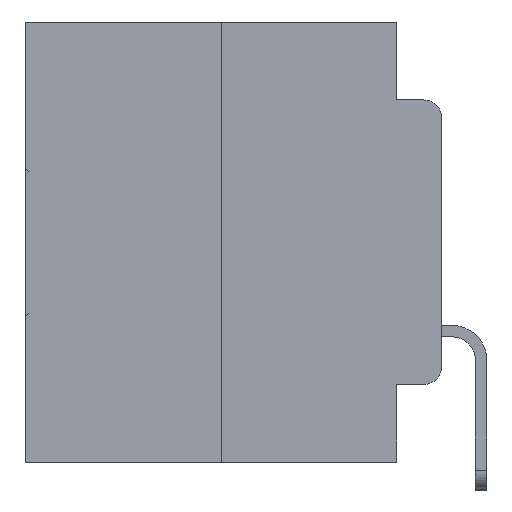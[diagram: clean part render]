
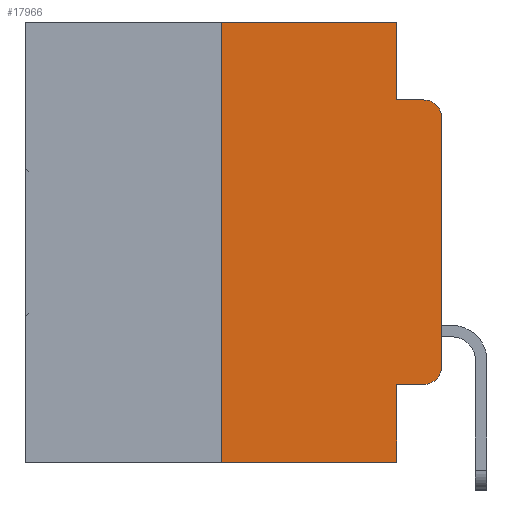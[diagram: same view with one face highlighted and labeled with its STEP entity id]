
A CAD part, left-side view. The second image highlights one B-rep face of the part: STEP entity #17966.
In plain terms, the highlighted planar face has unit normal (-1, 0, 0).
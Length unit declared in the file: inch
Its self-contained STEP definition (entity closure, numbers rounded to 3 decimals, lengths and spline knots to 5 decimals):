
#296 = EDGE_LOOP ( 'NONE', ( #29624, #25712, #14131, #27852, #28218, #24323, #12655, #25744, #20399, #16408 ) ) ;
#728 = CARTESIAN_POINT ( 'NONE',  ( 0., 0., 0. ) ) ;
#784 = LINE ( 'NONE', #728, #25386 ) ;
#1625 = EDGE_CURVE ( 'NONE', #17362, #16913, #1626, .T. ) ;
#1626 = CIRCLE ( 'NONE', #25151, 0.02 ) ;
#2465 = LINE ( 'NONE', #24249, #20825 ) ;
#2803 = CARTESIAN_POINT ( 'NONE',  ( 0., 0.473, -0.5 ) ) ;
#3307 = DIRECTION ( 'NONE',  ( 0., 0., 1. ) ) ;
#4111 = DIRECTION ( 'NONE',  ( 0., -1., 0. ) ) ;
#5017 = EDGE_CURVE ( 'NONE', #6628, #17362, #23708, .T. ) ;
#5331 = DIRECTION ( 'NONE',  ( 0., -1., 0. ) ) ;
#5444 = EDGE_CURVE ( 'NONE', #24147, #14313, #7922, .T. ) ;
#6575 = CARTESIAN_POINT ( 'NONE',  ( 0., 0.473, 0. ) ) ;
#6628 = VERTEX_POINT ( 'NONE', #30108 ) ;
#6694 = CARTESIAN_POINT ( 'NONE',  ( 0., 0., -0.3915 ) ) ;
#7062 = VECTOR ( 'NONE', #21141, 39.37008 ) ;
#7149 = VECTOR ( 'NONE', #5331, 39.37008 ) ;
#7552 = CARTESIAN_POINT ( 'NONE',  ( 0., 0.02, -0.3915 ) ) ;
#7922 = LINE ( 'NONE', #2803, #7149 ) ;
#8046 = LINE ( 'NONE', #6575, #25957 ) ;
#8290 = EDGE_CURVE ( 'NONE', #6628, #14313, #2465, .T. ) ;
#8490 = CARTESIAN_POINT ( 'NONE',  ( 0., 0.473, 0. ) ) ;
#8543 = CARTESIAN_POINT ( 'NONE',  ( 0., 0.25, 0. ) ) ;
#8690 = DIRECTION ( 'NONE',  ( -1., 0., 0. ) ) ;
#8736 = CARTESIAN_POINT ( 'NONE',  ( 0., 0.051, -0.4115 ) ) ;
#8825 = CARTESIAN_POINT ( 'NONE',  ( 0., 0.051, 0. ) ) ;
#9411 = CARTESIAN_POINT ( 'NONE',  ( 0., 0.02, -0.0885 ) ) ;
#11488 = EDGE_CURVE ( 'NONE', #24147, #15860, #26339, .T. ) ;
#11588 = LINE ( 'NONE', #19626, #29333 ) ;
#11715 = EDGE_CURVE ( 'NONE', #15860, #23258, #8046, .T. ) ;
#12637 = DIRECTION ( 'NONE',  ( 0., 0., -1. ) ) ;
#12655 = ORIENTED_EDGE ( 'NONE', *, *, #5444, .T. ) ;
#12989 = CARTESIAN_POINT ( 'NONE',  ( 0., 0.25, 0. ) ) ;
#13060 = CARTESIAN_POINT ( 'NONE',  ( 0., 0.02, -0.4115 ) ) ;
#13401 = DIRECTION ( 'NONE',  ( 0., 0., -1. ) ) ;
#14131 = ORIENTED_EDGE ( 'NONE', *, *, #17877, .F. ) ;
#14164 = LINE ( 'NONE', #23317, #7062 ) ;
#14313 = VERTEX_POINT ( 'NONE', #15365 ) ;
#14548 = DIRECTION ( 'NONE',  ( -1., 0., 0. ) ) ;
#14674 = EDGE_CURVE ( 'NONE', #23258, #28104, #14164, .T. ) ;
#15365 = CARTESIAN_POINT ( 'NONE',  ( 0., 0.051, -0.5 ) ) ;
#15860 = VERTEX_POINT ( 'NONE', #8543 ) ;
#16408 = ORIENTED_EDGE ( 'NONE', *, *, #1625, .T. ) ;
#16656 = AXIS2_PLACEMENT_3D ( 'NONE', #22754, #8690, #25051 ) ;
#16750 = CIRCLE ( 'NONE', #16656, 0.02 ) ;
#16913 = VERTEX_POINT ( 'NONE', #6694 ) ;
#17362 = VERTEX_POINT ( 'NONE', #13060 ) ;
#17652 = VECTOR ( 'NONE', #20610, 39.37008 ) ;
#17696 = VERTEX_POINT ( 'NONE', #9411 ) ;
#17814 = AXIS2_PLACEMENT_3D ( 'NONE', #8490, #27258, #13401 ) ;
#17877 = EDGE_CURVE ( 'NONE', #28104, #17696, #11588, .T. ) ;
#17966 = ADVANCED_FACE ( 'NONE', ( #27899 ), #22671, .F. ) ;
#19626 = CARTESIAN_POINT ( 'NONE',  ( 0., 0.051, -0.0885 ) ) ;
#20399 = ORIENTED_EDGE ( 'NONE', *, *, #5017, .T. ) ;
#20610 = DIRECTION ( 'NONE',  ( 0., -1., 0. ) ) ;
#20825 = VECTOR ( 'NONE', #12637, 39.37008 ) ;
#20934 = EDGE_CURVE ( 'NONE', #27438, #17696, #16750, .T. ) ;
#21141 = DIRECTION ( 'NONE',  ( 0., 0., -1. ) ) ;
#21931 = DIRECTION ( 'NONE',  ( 0., -1., 0. ) ) ;
#22467 = EDGE_CURVE ( 'NONE', #16913, #27438, #784, .T. ) ;
#22671 = PLANE ( 'NONE',  #17814 ) ;
#22754 = CARTESIAN_POINT ( 'NONE',  ( 0., 0.02, -0.1085 ) ) ;
#23258 = VERTEX_POINT ( 'NONE', #8825 ) ;
#23317 = CARTESIAN_POINT ( 'NONE',  ( 0., 0.051, 0. ) ) ;
#23571 = CARTESIAN_POINT ( 'NONE',  ( 0., 0., -0.1085 ) ) ;
#23708 = LINE ( 'NONE', #8736, #17652 ) ;
#23737 = CARTESIAN_POINT ( 'NONE',  ( 0., 0.051, -0.0885 ) ) ;
#24147 = VERTEX_POINT ( 'NONE', #30121 ) ;
#24249 = CARTESIAN_POINT ( 'NONE',  ( 0., 0.051, 0. ) ) ;
#24323 = ORIENTED_EDGE ( 'NONE', *, *, #11488, .F. ) ;
#24583 = DIRECTION ( 'NONE',  ( 0., 0., 1. ) ) ;
#25051 = DIRECTION ( 'NONE',  ( 0., 0., -1. ) ) ;
#25151 = AXIS2_PLACEMENT_3D ( 'NONE', #7552, #14548, #30622 ) ;
#25386 = VECTOR ( 'NONE', #3307, 39.37008 ) ;
#25618 = VECTOR ( 'NONE', #24583, 39.37008 ) ;
#25712 = ORIENTED_EDGE ( 'NONE', *, *, #20934, .T. ) ;
#25744 = ORIENTED_EDGE ( 'NONE', *, *, #8290, .F. ) ;
#25957 = VECTOR ( 'NONE', #4111, 39.37008 ) ;
#26339 = LINE ( 'NONE', #12989, #25618 ) ;
#27258 = DIRECTION ( 'NONE',  ( 1., 0., 0. ) ) ;
#27438 = VERTEX_POINT ( 'NONE', #23571 ) ;
#27852 = ORIENTED_EDGE ( 'NONE', *, *, #14674, .F. ) ;
#27899 = FACE_OUTER_BOUND ( 'NONE', #296, .T. ) ;
#28104 = VERTEX_POINT ( 'NONE', #23737 ) ;
#28218 = ORIENTED_EDGE ( 'NONE', *, *, #11715, .F. ) ;
#29333 = VECTOR ( 'NONE', #21931, 39.37008 ) ;
#29624 = ORIENTED_EDGE ( 'NONE', *, *, #22467, .T. ) ;
#30108 = CARTESIAN_POINT ( 'NONE',  ( 0., 0.051, -0.4115 ) ) ;
#30121 = CARTESIAN_POINT ( 'NONE',  ( 0., 0.25, -0.5 ) ) ;
#30622 = DIRECTION ( 'NONE',  ( 0., 0., -1. ) ) ;
